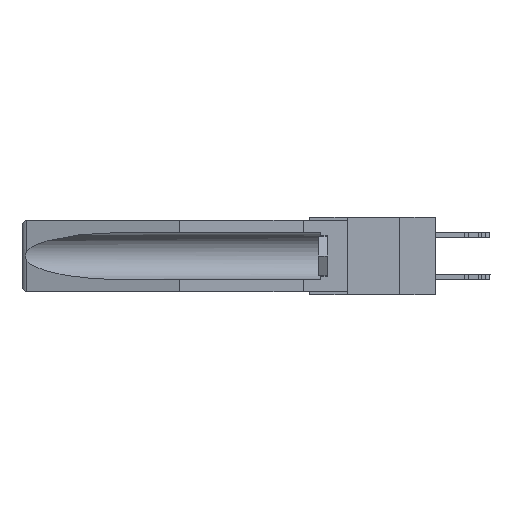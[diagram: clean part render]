
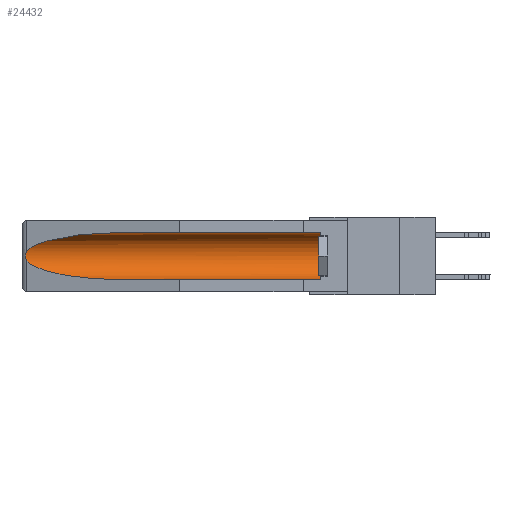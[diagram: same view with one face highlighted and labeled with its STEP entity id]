
A CAD part, left-side view. The second image highlights one B-rep face of the part: STEP entity #24432.
In plain terms, the highlighted cylindrical face has radius 2.857 mm (diameter 5.715 mm), a partial arc.
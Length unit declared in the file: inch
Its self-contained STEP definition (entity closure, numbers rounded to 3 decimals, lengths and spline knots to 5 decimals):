
#239 = ORIENTED_EDGE ( 'NONE', *, *, #9403, .T. ) ;
#931 = CARTESIAN_POINT ( 'NONE',  ( 0.26537, 1.52718, -0.19328 ) ) ;
#1145 = B_SPLINE_CURVE_WITH_KNOTS ( 'NONE', 3,
 ( #15163, #10306, #20317, #27388, #7746, #8070, #15059, #15257, #3197, #931 ),
 .UNSPECIFIED., .F., .F.,
 ( 4, 2, 2, 2, 4 ),
 ( 0., 0.00029, 0.00058, 0.00087, 0.00117 ),
 .UNSPECIFIED. ) ;
#1422 = CARTESIAN_POINT ( 'NONE',  ( 0.26537, 1.52718, -0.19328 ) ) ;
#1962 = VECTOR ( 'NONE', #20188, 39.37008 ) ;
#2192 = ORIENTED_EDGE ( 'NONE', *, *, #8895, .F. ) ;
#3197 = CARTESIAN_POINT ( 'NONE',  ( 0.26597, 1.5296, -0.19026 ) ) ;
#3419 = CARTESIAN_POINT ( 'NONE',  ( 0.155, -0.30754, -0.284 ) ) ;
#4292 = CARTESIAN_POINT ( 'NONE',  ( 0.155, 1.07973, -0.284 ) ) ;
#6387 = FACE_OUTER_BOUND ( 'NONE', #13366, .T. ) ;
#6772 = ORIENTED_EDGE ( 'NONE', *, *, #21770, .T. ) ;
#7045 = CARTESIAN_POINT ( 'NONE',  ( 0.155, 1.07973, -0.284 ) ) ;
#7088 = EDGE_CURVE ( 'NONE', #10476, #21543, #27250, .T. ) ;
#7746 = CARTESIAN_POINT ( 'NONE',  ( 0.2675, 1.53308, -0.16763 ) ) ;
#8070 = CARTESIAN_POINT ( 'NONE',  ( 0.2675, 1.53308, -0.17534 ) ) ;
#8492 = DIRECTION ( 'NONE',  ( 0., 0., 1. ) ) ;
#8895 = EDGE_CURVE ( 'NONE', #15444, #21543, #26173, .T. ) ;
#9064 = CARTESIAN_POINT ( 'NONE',  ( 0.155, 1.07973, -0.059 ) ) ;
#9403 = EDGE_CURVE ( 'NONE', #25288, #22536, #17808, .T. ) ;
#9487 = CYLINDRICAL_SURFACE ( 'NONE', #15037, 0.1125 ) ;
#10306 = CARTESIAN_POINT ( 'NONE',  ( 0.26597, 1.52961, -0.15275 ) ) ;
#10377 = CARTESIAN_POINT ( 'NONE',  ( 0.155, 0.126, -0.284 ) ) ;
#10476 = VERTEX_POINT ( 'NONE', #1422 ) ;
#10656 = ORIENTED_EDGE ( 'NONE', *, *, #7088, .T. ) ;
#11033 = DIRECTION ( 'NONE',  ( 0., 0., 1. ) ) ;
#11736 = ORIENTED_EDGE ( 'NONE', *, *, #25301, .T. ) ;
#13063 = CARTESIAN_POINT ( 'NONE',  ( 0.25451, 1.48313, -0.09465 ) ) ;
#13321 = VECTOR ( 'NONE', #13475, 39.37008 ) ;
#13359 = CARTESIAN_POINT ( 'NONE',  ( 0.155, 0.126, -0.1715 ) ) ;
#13366 = EDGE_LOOP ( 'NONE', ( #26033, #11736, #10656, #2192, #6772, #239 ) ) ;
#13475 = DIRECTION ( 'NONE',  ( 0., 1., 0. ) ) ;
#15037 = AXIS2_PLACEMENT_3D ( 'NONE', #30239, #15782, #11033 ) ;
#15059 = CARTESIAN_POINT ( 'NONE',  ( 0.2673, 1.53269, -0.17917 ) ) ;
#15163 = CARTESIAN_POINT ( 'NONE',  ( 0.26537, 1.52718, -0.14972 ) ) ;
#15257 = CARTESIAN_POINT ( 'NONE',  ( 0.26655, 1.53094, -0.18657 ) ) ;
#15444 = VERTEX_POINT ( 'NONE', #10377 ) ;
#15782 = DIRECTION ( 'NONE',  ( 0., 1., 0. ) ) ;
#16559 = CARTESIAN_POINT ( 'NONE',  ( 0.21114, 1.30732, -0.284 ) ) ;
#17808 = LINE ( 'NONE', #27274, #1962 ) ;
#18559 = CARTESIAN_POINT ( 'NONE',  ( 0.26537, 1.52718, -0.19328 ) ) ;
#19140 = CARTESIAN_POINT ( 'NONE',  ( 0.21114, 1.30732, -0.059 ) ) ;
#20188 = DIRECTION ( 'NONE',  ( 0., 1., 0. ) ) ;
#20317 = CARTESIAN_POINT ( 'NONE',  ( 0.26654, 1.53092, -0.15636 ) ) ;
#20535 = DIRECTION ( 'NONE',  ( 0., -1., 0. ) ) ;
#20615 = AXIS2_PLACEMENT_3D ( 'NONE', #13359, #20535, #8492 ) ;
#21543 = VERTEX_POINT ( 'NONE', #7045 ) ;
#21770 = EDGE_CURVE ( 'NONE', #15444, #25288, #28643, .T. ) ;
#22536 = VERTEX_POINT ( 'NONE', #9064 ) ;
#22657 = CARTESIAN_POINT ( 'NONE',  ( 0.155, 0.126, -0.059 ) ) ;
#23291 = CARTESIAN_POINT ( 'NONE',  ( 0.26537, 1.52718, -0.14972 ) ) ;
#23583 =( BOUNDED_CURVE ( )  B_SPLINE_CURVE ( 3, ( #26412, #19140, #13063, #27108 ),
 .UNSPECIFIED., .F., .F. ) 
 B_SPLINE_CURVE_WITH_KNOTS ( ( 4, 4 ),
 ( 4.71239, 6.08839 ),
 .UNSPECIFIED. ) 
 CURVE ( )  GEOMETRIC_REPRESENTATION_ITEM ( )  RATIONAL_B_SPLINE_CURVE ( ( 1., 0.848, 0.848, 1. ) ) 
 REPRESENTATION_ITEM ( '' )  );
#24432 = ADVANCED_FACE ( 'NONE', ( #6387 ), #9487, .F. ) ;
#25288 = VERTEX_POINT ( 'NONE', #22657 ) ;
#25301 = EDGE_CURVE ( 'NONE', #25534, #10476, #1145, .T. ) ;
#25534 = VERTEX_POINT ( 'NONE', #23291 ) ;
#26033 = ORIENTED_EDGE ( 'NONE', *, *, #27753, .T. ) ;
#26173 = LINE ( 'NONE', #3419, #13321 ) ;
#26412 = CARTESIAN_POINT ( 'NONE',  ( 0.155, 1.07973, -0.059 ) ) ;
#27108 = CARTESIAN_POINT ( 'NONE',  ( 0.26537, 1.52718, -0.14972 ) ) ;
#27250 =( BOUNDED_CURVE ( )  B_SPLINE_CURVE ( 3, ( #18559, #30785, #16559, #4292 ),
 .UNSPECIFIED., .F., .F. ) 
 B_SPLINE_CURVE_WITH_KNOTS ( ( 4, 4 ),
 ( 0.1948, 1.5708 ),
 .UNSPECIFIED. ) 
 CURVE ( )  GEOMETRIC_REPRESENTATION_ITEM ( )  RATIONAL_B_SPLINE_CURVE ( ( 1., 0.848, 0.848, 1. ) ) 
 REPRESENTATION_ITEM ( '' )  );
#27274 = CARTESIAN_POINT ( 'NONE',  ( 0.155, -0.30754, -0.059 ) ) ;
#27388 = CARTESIAN_POINT ( 'NONE',  ( 0.2673, 1.5327, -0.16383 ) ) ;
#27753 = EDGE_CURVE ( 'NONE', #22536, #25534, #23583, .T. ) ;
#28643 = CIRCLE ( 'NONE', #20615, 0.1125 ) ;
#30239 = CARTESIAN_POINT ( 'NONE',  ( 0.155, -0.30754, -0.1715 ) ) ;
#30785 = CARTESIAN_POINT ( 'NONE',  ( 0.25451, 1.48313, -0.24835 ) ) ;
